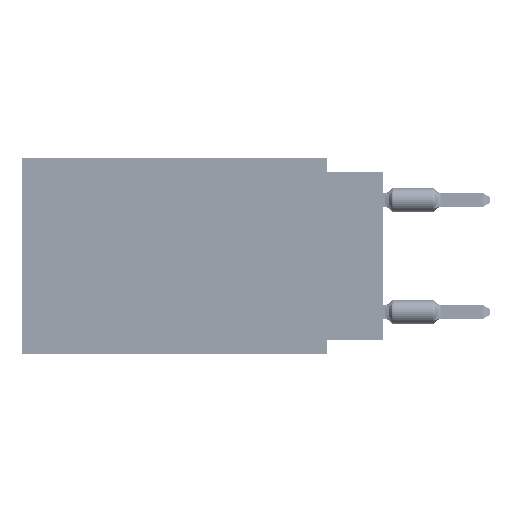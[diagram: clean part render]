
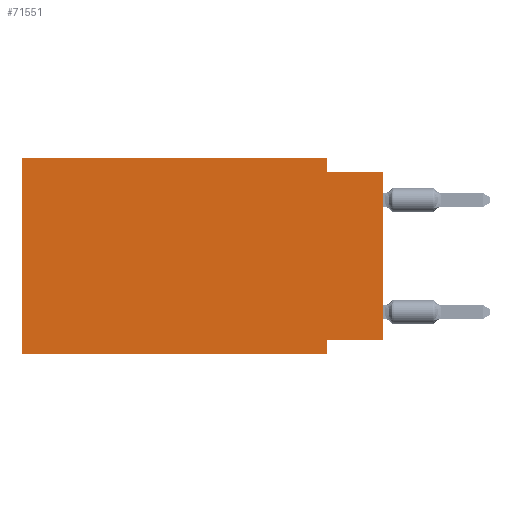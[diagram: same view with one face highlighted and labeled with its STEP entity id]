
A CAD part, left-side view. The second image highlights one B-rep face of the part: STEP entity #71551.
In plain terms, the highlighted planar face has unit normal (-1, 0, 0).
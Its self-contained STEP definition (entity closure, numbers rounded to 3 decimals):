
#4277 = VECTOR ( 'NONE', #54699, 1000. ) ;
#4446 = ORIENTED_EDGE ( 'NONE', *, *, #20315, .F. ) ;
#4807 = EDGE_CURVE ( 'NONE', #19648, #29440, #23723, .T. ) ;
#4922 = EDGE_CURVE ( 'NONE', #24471, #69201, #18803, .T. ) ;
#6116 = CARTESIAN_POINT ( 'NONE',  ( 0., 2.54, -8.89 ) ) ;
#6569 = DIRECTION ( 'NONE',  ( 0., 0., -1. ) ) ;
#7490 = VERTEX_POINT ( 'NONE', #43607 ) ;
#9792 = EDGE_LOOP ( 'NONE', ( #87140, #53926, #76106, #4446, #73245, #58994, #14599, #56654 ) ) ;
#10111 = EDGE_CURVE ( 'NONE', #30815, #7490, #46885, .T. ) ;
#10961 = CARTESIAN_POINT ( 'NONE',  ( 0., 0., -8.255 ) ) ;
#11037 = VECTOR ( 'NONE', #63537, 1000. ) ;
#11042 = VECTOR ( 'NONE', #6569, 1000. ) ;
#12296 = DIRECTION ( 'NONE',  ( 0., 0., 1. ) ) ;
#14599 = ORIENTED_EDGE ( 'NONE', *, *, #35081, .F. ) ;
#17058 = CARTESIAN_POINT ( 'NONE',  ( 0., 0., -8.255 ) ) ;
#18803 = LINE ( 'NONE', #86245, #27997 ) ;
#19648 = VERTEX_POINT ( 'NONE', #10961 ) ;
#20311 = LINE ( 'NONE', #6116, #11042 ) ;
#20315 = EDGE_CURVE ( 'NONE', #7490, #34499, #69324, .T. ) ;
#22491 = VECTOR ( 'NONE', #12296, 1000. ) ;
#23723 = LINE ( 'NONE', #17058, #60619 ) ;
#24471 = VERTEX_POINT ( 'NONE', #61777 ) ;
#24526 = VERTEX_POINT ( 'NONE', #68422 ) ;
#27633 = CARTESIAN_POINT ( 'NONE',  ( 0., 16.383, -8.89 ) ) ;
#27997 = VECTOR ( 'NONE', #32997, 1000. ) ;
#29440 = VERTEX_POINT ( 'NONE', #69800 ) ;
#30815 = VERTEX_POINT ( 'NONE', #69743 ) ;
#32670 = VECTOR ( 'NONE', #75263, 1000. ) ;
#32986 = LINE ( 'NONE', #27633, #4277 ) ;
#32997 = DIRECTION ( 'NONE',  ( 0., -1., 0. ) ) ;
#33570 = CARTESIAN_POINT ( 'NONE',  ( 0., 16.383, 0. ) ) ;
#33877 = EDGE_CURVE ( 'NONE', #34499, #24471, #47833, .T. ) ;
#34499 = VERTEX_POINT ( 'NONE', #43678 ) ;
#35081 = EDGE_CURVE ( 'NONE', #29440, #24526, #20311, .T. ) ;
#36657 = FACE_OUTER_BOUND ( 'NONE', #9792, .T. ) ;
#42859 = DIRECTION ( 'NONE',  ( 0., 0., -1. ) ) ;
#43111 = CARTESIAN_POINT ( 'NONE',  ( 0., 16.383, 0. ) ) ;
#43607 = CARTESIAN_POINT ( 'NONE',  ( 0., 16.383, 0. ) ) ;
#43678 = CARTESIAN_POINT ( 'NONE',  ( 0., 2.54, 0. ) ) ;
#44125 = DIRECTION ( 'NONE',  ( 0., 1., 0. ) ) ;
#46885 = LINE ( 'NONE', #33570, #32670 ) ;
#47390 = DIRECTION ( 'NONE',  ( 0., 0., -1. ) ) ;
#47833 = LINE ( 'NONE', #67365, #83407 ) ;
#47882 = EDGE_CURVE ( 'NONE', #19648, #69201, #52691, .T. ) ;
#52691 = LINE ( 'NONE', #79337, #22491 ) ;
#53926 = ORIENTED_EDGE ( 'NONE', *, *, #4922, .F. ) ;
#54699 = DIRECTION ( 'NONE',  ( 0., -1., 0. ) ) ;
#56654 = ORIENTED_EDGE ( 'NONE', *, *, #4807, .F. ) ;
#57497 = CARTESIAN_POINT ( 'NONE',  ( 0., 16.383, 0. ) ) ;
#58994 = ORIENTED_EDGE ( 'NONE', *, *, #67427, .T. ) ;
#60619 = VECTOR ( 'NONE', #44125, 1000. ) ;
#61777 = CARTESIAN_POINT ( 'NONE',  ( 0., 2.54, -0.635 ) ) ;
#63537 = DIRECTION ( 'NONE',  ( 0., -1., 0. ) ) ;
#63725 = PLANE ( 'NONE',  #71499 ) ;
#67365 = CARTESIAN_POINT ( 'NONE',  ( 0., 2.54, 0. ) ) ;
#67427 = EDGE_CURVE ( 'NONE', #30815, #24526, #32986, .T. ) ;
#68422 = CARTESIAN_POINT ( 'NONE',  ( 0., 2.54, -8.89 ) ) ;
#69201 = VERTEX_POINT ( 'NONE', #82987 ) ;
#69324 = LINE ( 'NONE', #43111, #11037 ) ;
#69743 = CARTESIAN_POINT ( 'NONE',  ( 0., 16.383, -8.89 ) ) ;
#69800 = CARTESIAN_POINT ( 'NONE',  ( 0., 2.54, -8.255 ) ) ;
#71499 = AXIS2_PLACEMENT_3D ( 'NONE', #57497, #84565, #42859 ) ;
#71551 = ADVANCED_FACE ( 'NONE', ( #36657 ), #63725, .F. ) ;
#73245 = ORIENTED_EDGE ( 'NONE', *, *, #10111, .F. ) ;
#75263 = DIRECTION ( 'NONE',  ( 0., 0., 1. ) ) ;
#76106 = ORIENTED_EDGE ( 'NONE', *, *, #33877, .F. ) ;
#79337 = CARTESIAN_POINT ( 'NONE',  ( 0., 0., 0. ) ) ;
#82987 = CARTESIAN_POINT ( 'NONE',  ( 0., 0., -0.635 ) ) ;
#83407 = VECTOR ( 'NONE', #47390, 1000. ) ;
#84565 = DIRECTION ( 'NONE',  ( 1., 0., 0. ) ) ;
#86245 = CARTESIAN_POINT ( 'NONE',  ( 0., 0., -0.635 ) ) ;
#87140 = ORIENTED_EDGE ( 'NONE', *, *, #47882, .T. ) ;
